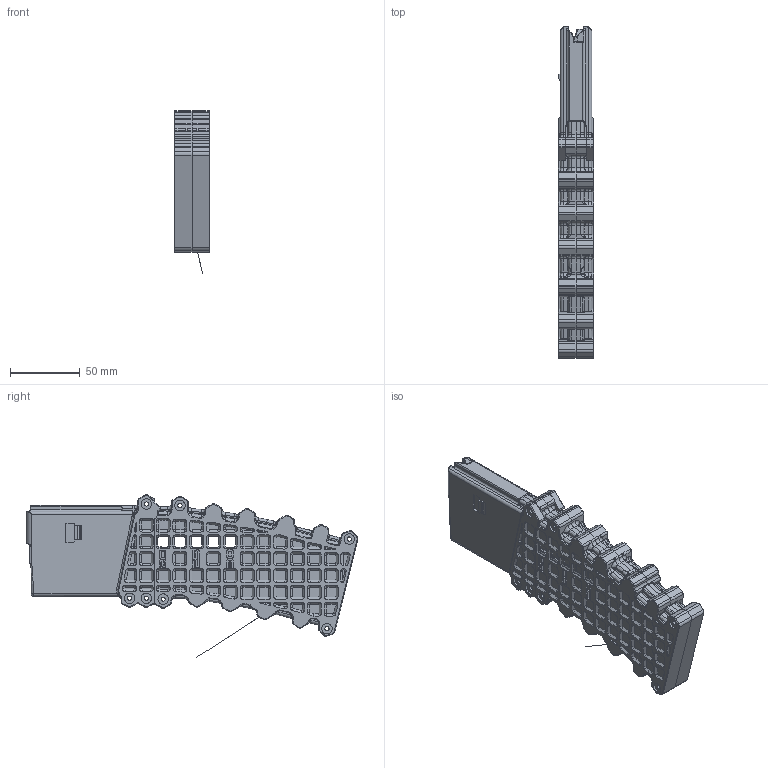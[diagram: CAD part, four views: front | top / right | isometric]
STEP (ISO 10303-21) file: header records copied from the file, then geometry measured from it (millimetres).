
FILE_DESCRIPTION (( 'STEP AP214' ), '1' );
FILE_NAME ('Extended Windowed Magazine.STEP', '2021-05-05T05:41:59', ( '' ), ( '' ), 'SwSTEP 2.0', 'SolidWorks 2020', '' );
FILE_SCHEMA (( 'AUTOMOTIVE_DESIGN' ));
Length unit declared in the file: millimetre
Products named in the file (5): Mag Follower; Extended Windowed Mag Body Bottom Right; Extended Windowed Mag Body Bottom Left; Mag Body Top; Extended Windowed Magazine
Assembly tree (4 placements, depth 2):
  Extended Windowed Magazine
    Mag Body Top
    Mag Follower
    Extended Windowed Mag Body Bottom Left
    Extended Windowed Mag Body Bottom Right
Bounding box: 25.5 x 237.2 x 116.14 mm (x, y, z)
Volume: 142869.7 mm3; surface area: 101229.6 mm2
Topology: 4 solids, 4 shells, 4227 faces, 10921 edges, 6732 vertices
Faces by surface type: plane 1373, cylinder 1041, bspline 876, cone 670, torus 224, sphere 43
Entity records: 161519 total; most frequent: CARTESIAN_POINT 64571, ORIENTED_EDGE 21562, DIRECTION 18616, EDGE_CURVE 10781, AXIS2_PLACEMENT_3D 6743, VERTEX_POINT 6723, LINE 5130, VECTOR 5130
